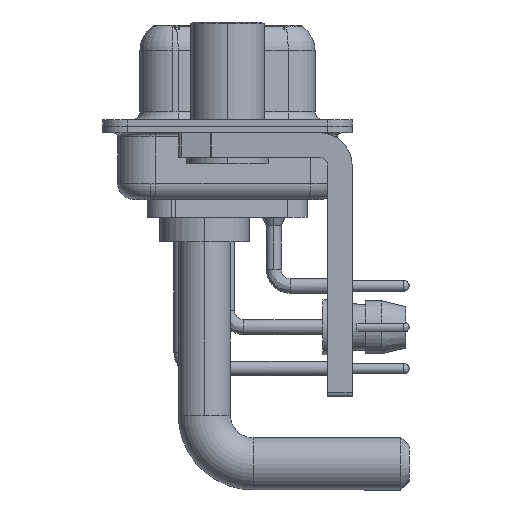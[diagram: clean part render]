
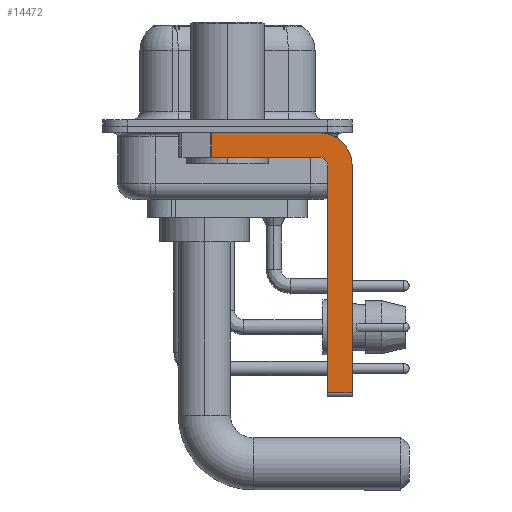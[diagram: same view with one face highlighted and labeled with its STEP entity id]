
A CAD part, left-side view. The second image highlights one B-rep face of the part: STEP entity #14472.
In plain terms, the highlighted planar face has unit normal (-1, 0, 0).
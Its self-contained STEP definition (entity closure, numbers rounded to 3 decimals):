
#589 = VERTEX_POINT ( 'NONE', #33519 ) ;
#633 = CIRCLE ( 'NONE', #27286, 2. ) ;
#2194 = CARTESIAN_POINT ( 'NONE',  ( -2.9, -5.65, -16.35 ) ) ;
#3194 = ORIENTED_EDGE ( 'NONE', *, *, #22964, .F. ) ;
#3353 = DIRECTION ( 'NONE',  ( 0., 0., -1. ) ) ;
#3531 = VECTOR ( 'NONE', #34861, 1000. ) ;
#5123 = CARTESIAN_POINT ( 'NONE',  ( -2.9, -7.65, -16.35 ) ) ;
#5874 = AXIS2_PLACEMENT_3D ( 'NONE', #24288, #24650, #10164 ) ;
#7022 = CARTESIAN_POINT ( 'NONE',  ( -2.9, -5.65, -1.9 ) ) ;
#7177 = ORIENTED_EDGE ( 'NONE', *, *, #9673, .T. ) ;
#7289 = DIRECTION ( 'NONE',  ( 1., 0., 0. ) ) ;
#7349 = ORIENTED_EDGE ( 'NONE', *, *, #12891, .F. ) ;
#7653 = EDGE_CURVE ( 'NONE', #17315, #23047, #33153, .T. ) ;
#8628 = LINE ( 'NONE', #22375, #30195 ) ;
#8897 = LINE ( 'NONE', #15363, #3531 ) ;
#9673 = EDGE_CURVE ( 'NONE', #21406, #35937, #8628, .T. ) ;
#9914 = ORIENTED_EDGE ( 'NONE', *, *, #10072, .F. ) ;
#10072 = EDGE_CURVE ( 'NONE', #21406, #589, #18443, .T. ) ;
#10164 = DIRECTION ( 'NONE',  ( 0., 0., 1. ) ) ;
#12040 = VECTOR ( 'NONE', #23605, 1000. ) ;
#12282 = CARTESIAN_POINT ( 'NONE',  ( -2.9, -6.15, -16.6 ) ) ;
#12891 = EDGE_CURVE ( 'NONE', #16148, #17315, #17328, .T. ) ;
#13505 = ORIENTED_EDGE ( 'NONE', *, *, #7653, .F. ) ;
#13710 = CARTESIAN_POINT ( 'NONE',  ( -2.9, 0.978, -1.9 ) ) ;
#14472 = ADVANCED_FACE ( 'NONE', ( #15626 ), #24184, .F. ) ;
#14962 = EDGE_CURVE ( 'NONE', #16148, #27825, #35974, .T. ) ;
#14992 = EDGE_LOOP ( 'NONE', ( #9914, #7177, #25342, #13505, #7349, #32024, #3194, #16178 ) ) ;
#15363 = CARTESIAN_POINT ( 'NONE',  ( -2.9, -5.65, -1.9 ) ) ;
#15598 = CARTESIAN_POINT ( 'NONE',  ( -2.9, -6.15, -16.35 ) ) ;
#15626 = FACE_OUTER_BOUND ( 'NONE', #14992, .T. ) ;
#16148 = VERTEX_POINT ( 'NONE', #15598 ) ;
#16178 = ORIENTED_EDGE ( 'NONE', *, *, #17171, .F. ) ;
#16376 = DIRECTION ( 'NONE',  ( 1., 0., 0. ) ) ;
#17171 = EDGE_CURVE ( 'NONE', #589, #26702, #633, .T. ) ;
#17315 = VERTEX_POINT ( 'NONE', #33868 ) ;
#17328 = LINE ( 'NONE', #12282, #12040 ) ;
#17821 = LINE ( 'NONE', #26351, #29327 ) ;
#18443 = LINE ( 'NONE', #27372, #18959 ) ;
#18959 = VECTOR ( 'NONE', #33114, 1000. ) ;
#19965 = DIRECTION ( 'NONE',  ( 0., 0., -1. ) ) ;
#21406 = VERTEX_POINT ( 'NONE', #27909 ) ;
#21977 = DIRECTION ( 'NONE',  ( 0., 0., -1. ) ) ;
#22375 = CARTESIAN_POINT ( 'NONE',  ( -2.9, 0.978, -1.9 ) ) ;
#22964 = EDGE_CURVE ( 'NONE', #26702, #27825, #17821, .T. ) ;
#23047 = VERTEX_POINT ( 'NONE', #7022 ) ;
#23605 = DIRECTION ( 'NONE',  ( 0., 0., 1. ) ) ;
#24184 = PLANE ( 'NONE',  #26486 ) ;
#24288 = CARTESIAN_POINT ( 'NONE',  ( -2.9, -5.65, -2.4 ) ) ;
#24650 = DIRECTION ( 'NONE',  ( -1., 0., 0. ) ) ;
#25342 = ORIENTED_EDGE ( 'NONE', *, *, #30989, .F. ) ;
#26351 = CARTESIAN_POINT ( 'NONE',  ( -2.9, -7.65, -2.4 ) ) ;
#26486 = AXIS2_PLACEMENT_3D ( 'NONE', #27357, #16376, #27716 ) ;
#26702 = VERTEX_POINT ( 'NONE', #34582 ) ;
#27286 = AXIS2_PLACEMENT_3D ( 'NONE', #27377, #7289, #21977 ) ;
#27357 = CARTESIAN_POINT ( 'NONE',  ( -2.9, -5.65, -2.4 ) ) ;
#27372 = CARTESIAN_POINT ( 'NONE',  ( -2.9, 3., -0.4 ) ) ;
#27377 = CARTESIAN_POINT ( 'NONE',  ( -2.9, -5.65, -2.4 ) ) ;
#27716 = DIRECTION ( 'NONE',  ( 0., 0., -1. ) ) ;
#27819 = DIRECTION ( 'NONE',  ( 0., -1., 0. ) ) ;
#27825 = VERTEX_POINT ( 'NONE', #5123 ) ;
#27909 = CARTESIAN_POINT ( 'NONE',  ( -2.9, 0.978, -0.4 ) ) ;
#29327 = VECTOR ( 'NONE', #3353, 1000. ) ;
#30195 = VECTOR ( 'NONE', #19965, 1000. ) ;
#30989 = EDGE_CURVE ( 'NONE', #23047, #35937, #8897, .T. ) ;
#32024 = ORIENTED_EDGE ( 'NONE', *, *, #14962, .T. ) ;
#33114 = DIRECTION ( 'NONE',  ( 0., -1., 0. ) ) ;
#33153 = CIRCLE ( 'NONE', #5874, 0.5 ) ;
#33519 = CARTESIAN_POINT ( 'NONE',  ( -2.9, -5.65, -0.4 ) ) ;
#33868 = CARTESIAN_POINT ( 'NONE',  ( -2.9, -6.15, -2.4 ) ) ;
#34264 = VECTOR ( 'NONE', #27819, 1000. ) ;
#34582 = CARTESIAN_POINT ( 'NONE',  ( -2.9, -7.65, -2.4 ) ) ;
#34861 = DIRECTION ( 'NONE',  ( 0., 1., 0. ) ) ;
#35937 = VERTEX_POINT ( 'NONE', #13710 ) ;
#35974 = LINE ( 'NONE', #2194, #34264 ) ;
